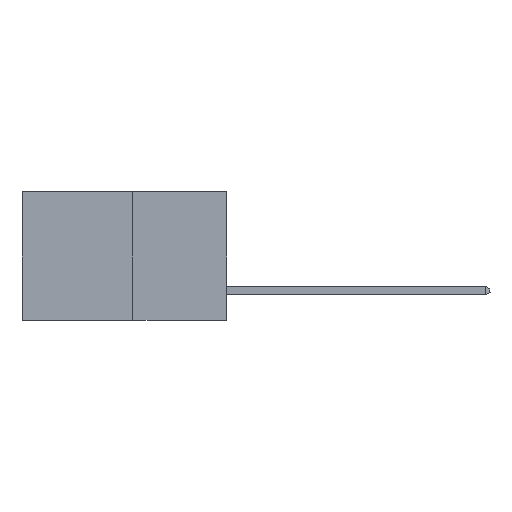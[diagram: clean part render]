
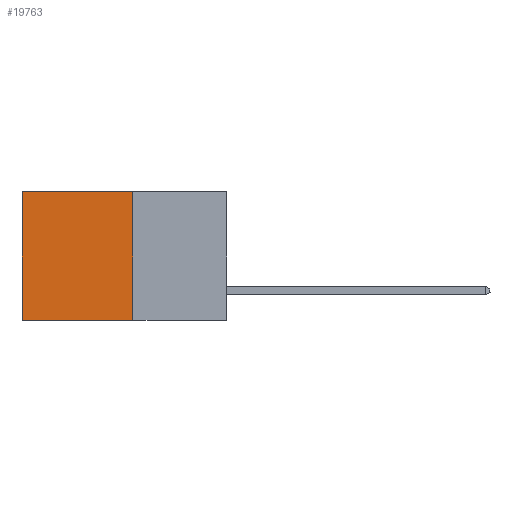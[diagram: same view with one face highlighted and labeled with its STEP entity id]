
A CAD part, left-side view. The second image highlights one B-rep face of the part: STEP entity #19763.
In plain terms, the highlighted planar face has unit normal (-1, 0, 0).
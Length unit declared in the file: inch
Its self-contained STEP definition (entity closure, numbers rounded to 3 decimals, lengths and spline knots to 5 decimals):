
#502 = LINE ( 'NONE', #8697, #15702 ) ;
#1167 = VECTOR ( 'NONE', #7559, 39.37008 ) ;
#1918 = EDGE_CURVE ( 'NONE', #4805, #25176, #8918, .T. ) ;
#2731 = PLANE ( 'NONE',  #13802 ) ;
#4078 = CARTESIAN_POINT ( 'NONE',  ( 0.277, 0.27, -0.37 ) ) ;
#4805 = VERTEX_POINT ( 'NONE', #18039 ) ;
#4892 = DIRECTION ( 'NONE',  ( 1., 0., 0. ) ) ;
#5848 = VECTOR ( 'NONE', #23508, 39.37008 ) ;
#6997 = ORIENTED_EDGE ( 'NONE', *, *, #1918, .T. ) ;
#7559 = DIRECTION ( 'NONE',  ( 0., 0., -1. ) ) ;
#8697 = CARTESIAN_POINT ( 'NONE',  ( 0.277, 0.27, -0.37 ) ) ;
#8918 = LINE ( 'NONE', #15991, #19746 ) ;
#11270 = LINE ( 'NONE', #18428, #1167 ) ;
#11721 = CARTESIAN_POINT ( 'NONE',  ( 0.277, 0.59, -0.37 ) ) ;
#13007 = ORIENTED_EDGE ( 'NONE', *, *, #25425, .F. ) ;
#13606 = VERTEX_POINT ( 'NONE', #4078 ) ;
#13802 = AXIS2_PLACEMENT_3D ( 'NONE', #22043, #4892, #20003 ) ;
#15393 = CARTESIAN_POINT ( 'NONE',  ( 0.277, 0.59, 0. ) ) ;
#15702 = VECTOR ( 'NONE', #19469, 39.37008 ) ;
#15881 = DIRECTION ( 'NONE',  ( 0., 1., 0. ) ) ;
#15991 = CARTESIAN_POINT ( 'NONE',  ( 0.277, 0.27, 0. ) ) ;
#17153 = EDGE_CURVE ( 'NONE', #13606, #24208, #502, .T. ) ;
#17652 = ORIENTED_EDGE ( 'NONE', *, *, #18828, .T. ) ;
#17677 = ORIENTED_EDGE ( 'NONE', *, *, #17153, .F. ) ;
#18039 = CARTESIAN_POINT ( 'NONE',  ( 0.277, 0.27, 0. ) ) ;
#18428 = CARTESIAN_POINT ( 'NONE',  ( 0.277, 0.27, -0.37 ) ) ;
#18828 = EDGE_CURVE ( 'NONE', #25176, #24208, #22351, .T. ) ;
#19469 = DIRECTION ( 'NONE',  ( 0., 1., 0. ) ) ;
#19746 = VECTOR ( 'NONE', #15881, 39.37008 ) ;
#19763 = ADVANCED_FACE ( 'NONE', ( #22206 ), #2731, .F. ) ;
#20003 = DIRECTION ( 'NONE',  ( 0., 0., -1. ) ) ;
#21432 = CARTESIAN_POINT ( 'NONE',  ( 0.277, 0.59, -0.37 ) ) ;
#22043 = CARTESIAN_POINT ( 'NONE',  ( 0.277, 0.27, -0.37 ) ) ;
#22206 = FACE_OUTER_BOUND ( 'NONE', #24595, .T. ) ;
#22351 = LINE ( 'NONE', #21432, #5848 ) ;
#23508 = DIRECTION ( 'NONE',  ( 0., 0., -1. ) ) ;
#24208 = VERTEX_POINT ( 'NONE', #11721 ) ;
#24595 = EDGE_LOOP ( 'NONE', ( #17652, #17677, #13007, #6997 ) ) ;
#25176 = VERTEX_POINT ( 'NONE', #15393 ) ;
#25425 = EDGE_CURVE ( 'NONE', #4805, #13606, #11270, .T. ) ;
